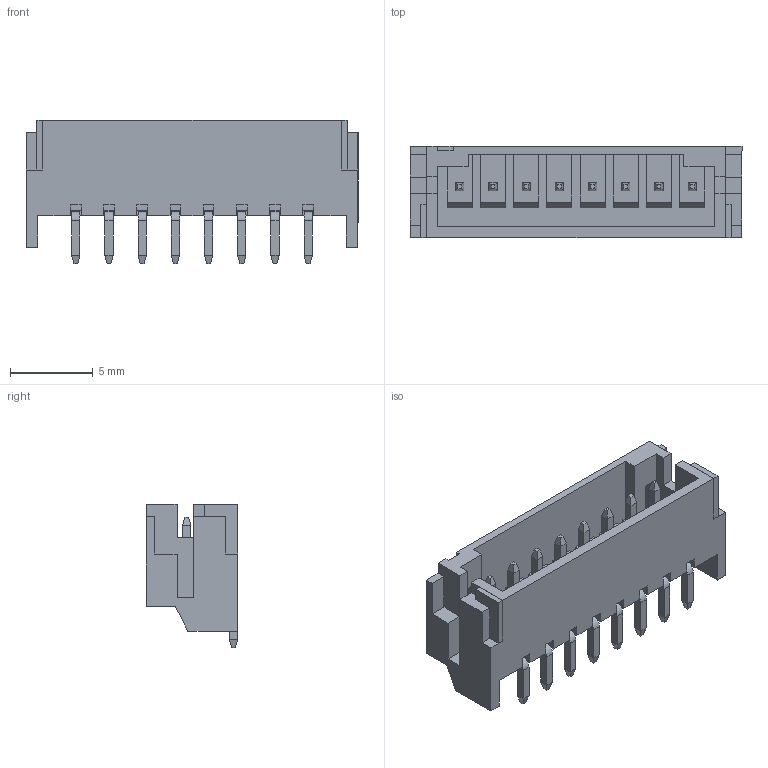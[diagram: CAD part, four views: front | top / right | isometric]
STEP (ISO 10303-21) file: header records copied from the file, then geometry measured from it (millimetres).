
FILE_DESCRIPTION (( 'STEP AP203' ), '1' );
FILE_NAME ('140-508-417-060.STEP', '2020-03-31T20:22:10', ( '' ), ( '' ), 'SwSTEP 2.0', 'SolidWorks 2016', '' );
FILE_SCHEMA (( 'CONFIG_CONTROL_DESIGN' ));
Length unit declared in the file: millimetre
Products named in the file (4): RA SMT Housing_508; RA SMT Pad; 140-508-417-060; RA SMT Contact
Assembly tree (11 placements, depth 2):
  140-508-417-060
    RA SMT Housing_508
    RA SMT Contact  x8
    RA SMT Pad  x2
Bounding box: 20 x 5.5 x 8.65 mm (x, y, z)
Volume: 281.4 mm3; surface area: 1048.5 mm2
Topology: 11 solids, 11 shells, 448 faces, 1096 edges, 666 vertices
Faces by surface type: plane 416, cylinder 32
Entity records: 8098 total; most frequent: CARTESIAN_POINT 1344, ORIENTED_EDGE 1328, DIRECTION 1164, EDGE_CURVE 664, VECTOR 656, LINE 656, VERTEX_POINT 434, AXIS2_PLACEMENT_3D 254
